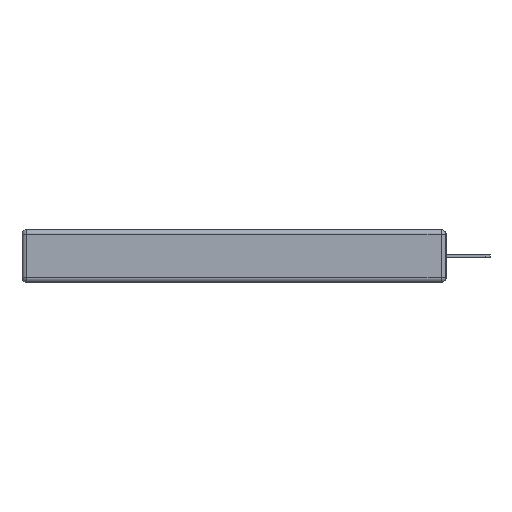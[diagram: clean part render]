
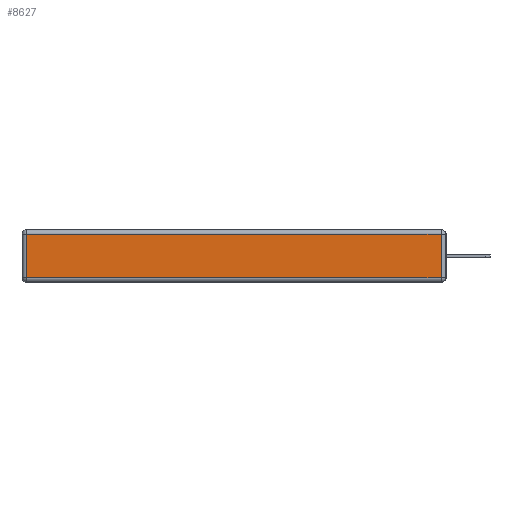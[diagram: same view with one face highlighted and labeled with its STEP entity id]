
A CAD part, left-side view. The second image highlights one B-rep face of the part: STEP entity #8627.
In plain terms, the highlighted planar face has unit normal (-1, 0, 0).
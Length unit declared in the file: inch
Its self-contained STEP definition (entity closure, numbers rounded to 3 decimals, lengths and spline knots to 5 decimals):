
#152 = CARTESIAN_POINT ( 'NONE',  ( 0., 2.72, -0.343 ) ) ;
#723 = EDGE_LOOP ( 'NONE', ( #13916, #3443, #3051, #15843 ) ) ;
#1082 = CARTESIAN_POINT ( 'NONE',  ( 0., 0., -0.313 ) ) ;
#1676 = CARTESIAN_POINT ( 'NONE',  ( 0., 2.72, -0.03 ) ) ;
#1822 = DIRECTION ( 'NONE',  ( 0., 0., 1. ) ) ;
#2124 = VERTEX_POINT ( 'NONE', #6064 ) ;
#2201 = VECTOR ( 'NONE', #14894, 39.37008 ) ;
#2708 = LINE ( 'NONE', #152, #9609 ) ;
#3034 = PLANE ( 'NONE',  #6946 ) ;
#3051 = ORIENTED_EDGE ( 'NONE', *, *, #10521, .T. ) ;
#3122 = CARTESIAN_POINT ( 'NONE',  ( 0., 0., -0.343 ) ) ;
#3252 = CARTESIAN_POINT ( 'NONE',  ( 0., 2.72, -0.313 ) ) ;
#3443 = ORIENTED_EDGE ( 'NONE', *, *, #9709, .T. ) ;
#3501 = EDGE_CURVE ( 'NONE', #13755, #2124, #13784, .T. ) ;
#3781 = VERTEX_POINT ( 'NONE', #5818 ) ;
#5818 = CARTESIAN_POINT ( 'NONE',  ( 0., 0.03, -0.03 ) ) ;
#6064 = CARTESIAN_POINT ( 'NONE',  ( 0., 0.03, -0.313 ) ) ;
#6504 = VECTOR ( 'NONE', #15200, 39.37008 ) ;
#6946 = AXIS2_PLACEMENT_3D ( 'NONE', #3122, #8152, #14263 ) ;
#8152 = DIRECTION ( 'NONE',  ( -1., 0., 0. ) ) ;
#8465 = EDGE_CURVE ( 'NONE', #14924, #13755, #2708, .T. ) ;
#8627 = ADVANCED_FACE ( 'NONE', ( #15505 ), #3034, .T. ) ;
#9609 = VECTOR ( 'NONE', #15261, 39.37008 ) ;
#9709 = EDGE_CURVE ( 'NONE', #2124, #3781, #13209, .T. ) ;
#10521 = EDGE_CURVE ( 'NONE', #3781, #14924, #16053, .T. ) ;
#12293 = CARTESIAN_POINT ( 'NONE',  ( 0., 2.75, -0.03 ) ) ;
#13039 = VECTOR ( 'NONE', #1822, 39.37008 ) ;
#13209 = LINE ( 'NONE', #14471, #13039 ) ;
#13755 = VERTEX_POINT ( 'NONE', #3252 ) ;
#13784 = LINE ( 'NONE', #1082, #6504 ) ;
#13916 = ORIENTED_EDGE ( 'NONE', *, *, #3501, .T. ) ;
#14263 = DIRECTION ( 'NONE',  ( 0., 0., 1. ) ) ;
#14471 = CARTESIAN_POINT ( 'NONE',  ( 0., 0.03, -0.343 ) ) ;
#14894 = DIRECTION ( 'NONE',  ( 0., 1., 0. ) ) ;
#14924 = VERTEX_POINT ( 'NONE', #1676 ) ;
#15200 = DIRECTION ( 'NONE',  ( 0., -1., 0. ) ) ;
#15261 = DIRECTION ( 'NONE',  ( 0., 0., -1. ) ) ;
#15505 = FACE_OUTER_BOUND ( 'NONE', #723, .T. ) ;
#15843 = ORIENTED_EDGE ( 'NONE', *, *, #8465, .T. ) ;
#16053 = LINE ( 'NONE', #12293, #2201 ) ;
